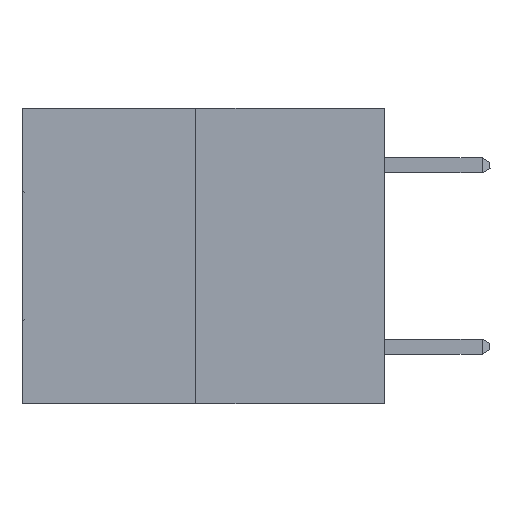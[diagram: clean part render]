
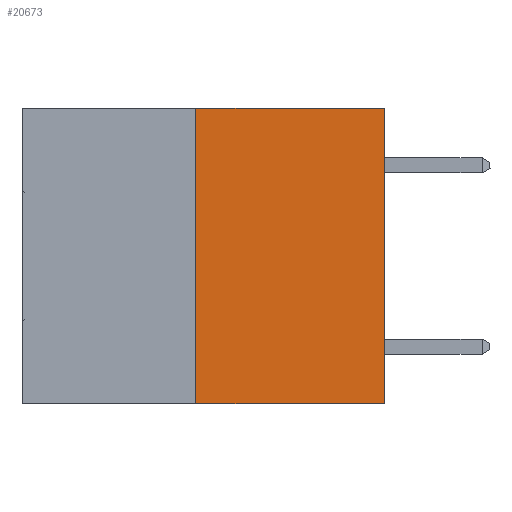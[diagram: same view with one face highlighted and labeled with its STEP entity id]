
A CAD part, left-side view. The second image highlights one B-rep face of the part: STEP entity #20673.
In plain terms, the highlighted planar face has unit normal (-1, 0, 0).
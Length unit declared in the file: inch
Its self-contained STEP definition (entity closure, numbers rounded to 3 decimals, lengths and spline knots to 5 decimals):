
#1886 = ORIENTED_EDGE ( 'NONE', *, *, #15895, .T. ) ;
#2400 = VECTOR ( 'NONE', #21159, 39.37008 ) ;
#3824 = DIRECTION ( 'NONE',  ( 0., 0., 1. ) ) ;
#4911 = DIRECTION ( 'NONE',  ( 0., 0., -1. ) ) ;
#6027 = CARTESIAN_POINT ( 'NONE',  ( 0., 0.6, -0.49 ) ) ;
#6105 = LINE ( 'NONE', #6027, #17886 ) ;
#6148 = EDGE_CURVE ( 'NONE', #8004, #30212, #7926, .T. ) ;
#6472 = CARTESIAN_POINT ( 'NONE',  ( 0., 0., 0. ) ) ;
#7693 = CARTESIAN_POINT ( 'NONE',  ( 0., 0.6, 0. ) ) ;
#7926 = LINE ( 'NONE', #7693, #2400 ) ;
#8004 = VERTEX_POINT ( 'NONE', #12276 ) ;
#9470 = EDGE_LOOP ( 'NONE', ( #27260, #1886, #11799, #23868 ) ) ;
#10729 = DIRECTION ( 'NONE',  ( 1., 0., 0. ) ) ;
#10884 = AXIS2_PLACEMENT_3D ( 'NONE', #34872, #10729, #4911 ) ;
#11799 = ORIENTED_EDGE ( 'NONE', *, *, #14663, .T. ) ;
#12276 = CARTESIAN_POINT ( 'NONE',  ( 0., 0.312, 0. ) ) ;
#13263 = DIRECTION ( 'NONE',  ( 0., 0., 1. ) ) ;
#14425 = VECTOR ( 'NONE', #13263, 39.37008 ) ;
#14663 = EDGE_CURVE ( 'NONE', #19023, #30212, #33131, .T. ) ;
#15895 = EDGE_CURVE ( 'NONE', #29715, #19023, #6105, .T. ) ;
#15924 = CARTESIAN_POINT ( 'NONE',  ( 0., 0., -0.49 ) ) ;
#17537 = CARTESIAN_POINT ( 'NONE',  ( 0., 0.312, -0.49 ) ) ;
#17886 = VECTOR ( 'NONE', #24886, 39.37008 ) ;
#18442 = EDGE_CURVE ( 'NONE', #29715, #8004, #23199, .T. ) ;
#19023 = VERTEX_POINT ( 'NONE', #15924 ) ;
#20673 = ADVANCED_FACE ( 'NONE', ( #21330 ), #34644, .F. ) ;
#21159 = DIRECTION ( 'NONE',  ( 0., -1., 0. ) ) ;
#21330 = FACE_OUTER_BOUND ( 'NONE', #9470, .T. ) ;
#23199 = LINE ( 'NONE', #17537, #23593 ) ;
#23593 = VECTOR ( 'NONE', #3824, 39.37008 ) ;
#23629 = CARTESIAN_POINT ( 'NONE',  ( 0., 0.312, -0.49 ) ) ;
#23868 = ORIENTED_EDGE ( 'NONE', *, *, #6148, .F. ) ;
#24886 = DIRECTION ( 'NONE',  ( 0., -1., 0. ) ) ;
#27260 = ORIENTED_EDGE ( 'NONE', *, *, #18442, .F. ) ;
#29715 = VERTEX_POINT ( 'NONE', #23629 ) ;
#30212 = VERTEX_POINT ( 'NONE', #6472 ) ;
#32094 = CARTESIAN_POINT ( 'NONE',  ( 0., 0., 0. ) ) ;
#33131 = LINE ( 'NONE', #32094, #14425 ) ;
#34644 = PLANE ( 'NONE',  #10884 ) ;
#34872 = CARTESIAN_POINT ( 'NONE',  ( 0., 0.6, 0. ) ) ;
